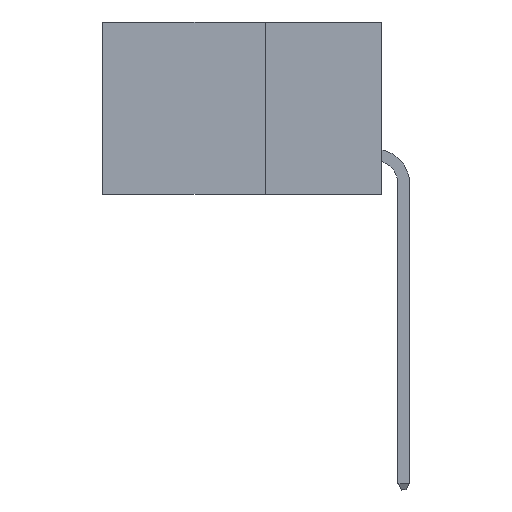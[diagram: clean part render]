
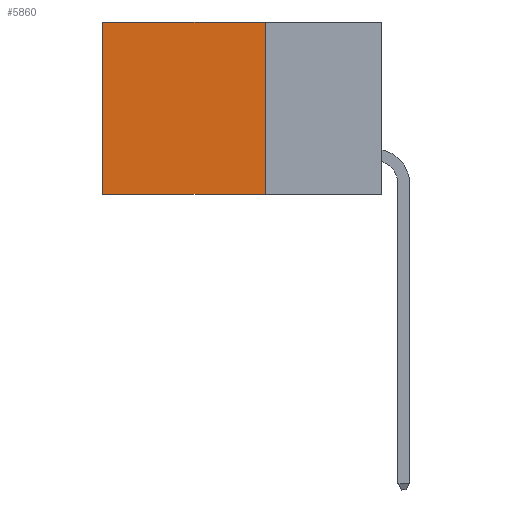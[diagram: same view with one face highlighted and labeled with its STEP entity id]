
A CAD part, left-side view. The second image highlights one B-rep face of the part: STEP entity #5860.
In plain terms, the highlighted planar face has unit normal (-1, 0, 0).
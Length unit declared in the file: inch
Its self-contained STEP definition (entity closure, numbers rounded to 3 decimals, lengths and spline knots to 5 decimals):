
#443 = VECTOR ( 'NONE', #9645, 39.37008 ) ;
#584 = DIRECTION ( 'NONE',  ( 0., 1., 0. ) ) ;
#686 = LINE ( 'NONE', #7897, #2509 ) ;
#1172 = ORIENTED_EDGE ( 'NONE', *, *, #8931, .T. ) ;
#1262 = CARTESIAN_POINT ( 'NONE',  ( 0.2875, 0.6, -0.37 ) ) ;
#2096 = VERTEX_POINT ( 'NONE', #5328 ) ;
#2406 = VECTOR ( 'NONE', #584, 39.37008 ) ;
#2509 = VECTOR ( 'NONE', #8927, 39.37008 ) ;
#2577 = EDGE_CURVE ( 'NONE', #4284, #11498, #686, .T. ) ;
#2789 = CARTESIAN_POINT ( 'NONE',  ( 0.2875, 0.25, 0. ) ) ;
#2868 = DIRECTION ( 'NONE',  ( 0., 0., -1. ) ) ;
#3605 = EDGE_CURVE ( 'NONE', #4335, #4284, #4358, .T. ) ;
#3933 = VECTOR ( 'NONE', #2868, 39.37008 ) ;
#4284 = VERTEX_POINT ( 'NONE', #6273 ) ;
#4310 = ORIENTED_EDGE ( 'NONE', *, *, #2577, .F. ) ;
#4335 = VERTEX_POINT ( 'NONE', #7117 ) ;
#4358 = LINE ( 'NONE', #2789, #3933 ) ;
#4713 = CARTESIAN_POINT ( 'NONE',  ( 0.2875, 0.25, 0. ) ) ;
#4757 = PLANE ( 'NONE',  #5915 ) ;
#5328 = CARTESIAN_POINT ( 'NONE',  ( 0.2875, 0.6, 0. ) ) ;
#5674 = DIRECTION ( 'NONE',  ( 0., 0., -1. ) ) ;
#5813 = CARTESIAN_POINT ( 'NONE',  ( 0.2875, 0.25, 0. ) ) ;
#5860 = ADVANCED_FACE ( 'NONE', ( #8627 ), #4757, .F. ) ;
#5915 = AXIS2_PLACEMENT_3D ( 'NONE', #4713, #11205, #5674 ) ;
#6273 = CARTESIAN_POINT ( 'NONE',  ( 0.2875, 0.25, -0.37 ) ) ;
#6602 = ORIENTED_EDGE ( 'NONE', *, *, #3605, .F. ) ;
#7117 = CARTESIAN_POINT ( 'NONE',  ( 0.2875, 0.25, 0. ) ) ;
#7897 = CARTESIAN_POINT ( 'NONE',  ( 0.2875, 0.25, -0.37 ) ) ;
#8627 = FACE_OUTER_BOUND ( 'NONE', #8640, .T. ) ;
#8640 = EDGE_LOOP ( 'NONE', ( #11468, #4310, #6602, #1172 ) ) ;
#8722 = EDGE_CURVE ( 'NONE', #2096, #11498, #10449, .T. ) ;
#8828 = CARTESIAN_POINT ( 'NONE',  ( 0.2875, 0.6, 0. ) ) ;
#8927 = DIRECTION ( 'NONE',  ( 0., 1., 0. ) ) ;
#8931 = EDGE_CURVE ( 'NONE', #4335, #2096, #10292, .T. ) ;
#9645 = DIRECTION ( 'NONE',  ( 0., 0., -1. ) ) ;
#10292 = LINE ( 'NONE', #5813, #2406 ) ;
#10449 = LINE ( 'NONE', #8828, #443 ) ;
#11205 = DIRECTION ( 'NONE',  ( 1., 0., 0. ) ) ;
#11468 = ORIENTED_EDGE ( 'NONE', *, *, #8722, .T. ) ;
#11498 = VERTEX_POINT ( 'NONE', #1262 ) ;
